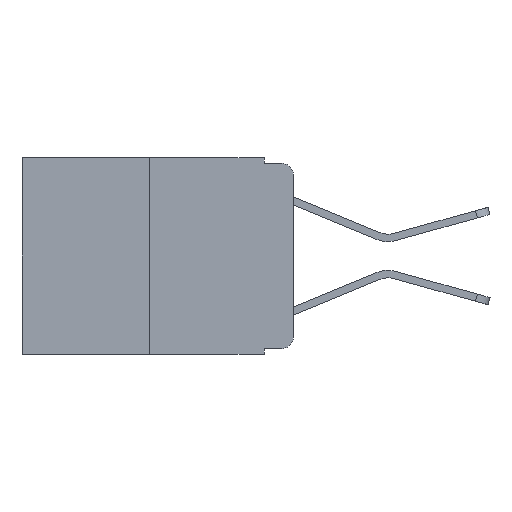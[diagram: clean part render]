
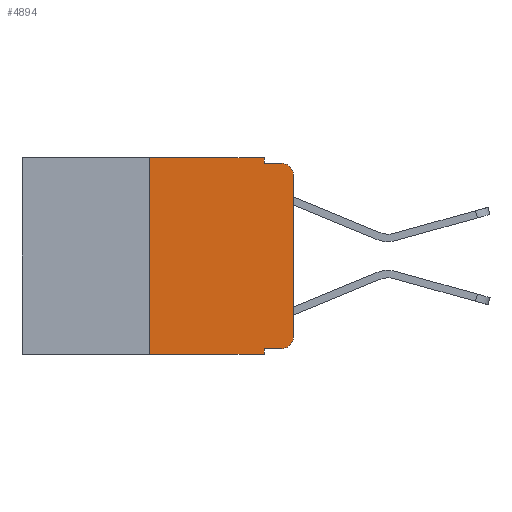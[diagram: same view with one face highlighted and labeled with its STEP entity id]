
A CAD part, left-side view. The second image highlights one B-rep face of the part: STEP entity #4894.
In plain terms, the highlighted planar face has unit normal (-1, 0, 0).
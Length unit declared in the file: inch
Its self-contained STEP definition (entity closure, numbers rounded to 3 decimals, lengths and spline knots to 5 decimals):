
#77 = CARTESIAN_POINT ( 'NONE',  ( 0., 0.02, -0.313 ) ) ;
#175 = VERTEX_POINT ( 'NONE', #5440 ) ;
#481 = FACE_OUTER_BOUND ( 'NONE', #11245, .T. ) ;
#937 = LINE ( 'NONE', #13470, #8280 ) ;
#971 = EDGE_CURVE ( 'NONE', #6619, #3720, #5943, .T. ) ;
#1068 = LINE ( 'NONE', #15789, #8590 ) ;
#1613 = ORIENTED_EDGE ( 'NONE', *, *, #971, .F. ) ;
#1691 = EDGE_CURVE ( 'NONE', #15083, #6226, #8127, .T. ) ;
#1909 = VERTEX_POINT ( 'NONE', #13209 ) ;
#2185 = ORIENTED_EDGE ( 'NONE', *, *, #8468, .T. ) ;
#2215 = CARTESIAN_POINT ( 'NONE',  ( 0., 0.051, -0.01 ) ) ;
#2357 = DIRECTION ( 'NONE',  ( 0., 0., -1. ) ) ;
#2562 = AXIS2_PLACEMENT_3D ( 'NONE', #15297, #12859, #10260 ) ;
#2727 = ORIENTED_EDGE ( 'NONE', *, *, #1691, .F. ) ;
#3245 = CIRCLE ( 'NONE', #2562, 0.02 ) ;
#3363 = ORIENTED_EDGE ( 'NONE', *, *, #11641, .T. ) ;
#3483 = DIRECTION ( 'NONE',  ( 1., 0., 0. ) ) ;
#3720 = VERTEX_POINT ( 'NONE', #12724 ) ;
#3867 = ORIENTED_EDGE ( 'NONE', *, *, #4759, .T. ) ;
#4334 = LINE ( 'NONE', #9506, #16254 ) ;
#4454 = PLANE ( 'NONE',  #15577 ) ;
#4559 = CARTESIAN_POINT ( 'NONE',  ( 0., 0.25, 0. ) ) ;
#4759 = EDGE_CURVE ( 'NONE', #8461, #175, #13996, .T. ) ;
#4894 = ADVANCED_FACE ( 'NONE', ( #481 ), #4454, .F. ) ;
#5097 = CARTESIAN_POINT ( 'NONE',  ( 0., 0.051, 0. ) ) ;
#5440 = CARTESIAN_POINT ( 'NONE',  ( 0., 0., -0.313 ) ) ;
#5709 = VECTOR ( 'NONE', #12184, 39.37008 ) ;
#5878 = LINE ( 'NONE', #9819, #7857 ) ;
#5943 = LINE ( 'NONE', #10983, #8694 ) ;
#6226 = VERTEX_POINT ( 'NONE', #2215 ) ;
#6250 = ORIENTED_EDGE ( 'NONE', *, *, #12152, .F. ) ;
#6619 = VERTEX_POINT ( 'NONE', #6769 ) ;
#6769 = CARTESIAN_POINT ( 'NONE',  ( 0., 0.051, -0.333 ) ) ;
#6835 = DIRECTION ( 'NONE',  ( 0., -1., 0. ) ) ;
#7012 = DIRECTION ( 'NONE',  ( 0., 0., -1. ) ) ;
#7691 = EDGE_CURVE ( 'NONE', #1909, #10425, #4334, .T. ) ;
#7712 = DIRECTION ( 'NONE',  ( -1., 0., 0. ) ) ;
#7757 = CARTESIAN_POINT ( 'NONE',  ( 0., 0.051, 0. ) ) ;
#7857 = VECTOR ( 'NONE', #16244, 39.37008 ) ;
#8127 = LINE ( 'NONE', #5097, #13311 ) ;
#8280 = VECTOR ( 'NONE', #9340, 39.37008 ) ;
#8325 = DIRECTION ( 'NONE',  ( 0., 0., 1. ) ) ;
#8424 = CARTESIAN_POINT ( 'NONE',  ( 0., 0.051, -0.333 ) ) ;
#8461 = VERTEX_POINT ( 'NONE', #9875 ) ;
#8468 = EDGE_CURVE ( 'NONE', #175, #11134, #5878, .T. ) ;
#8590 = VECTOR ( 'NONE', #6835, 39.37008 ) ;
#8694 = VECTOR ( 'NONE', #7012, 39.37008 ) ;
#9340 = DIRECTION ( 'NONE',  ( 0., -1., 0. ) ) ;
#9506 = CARTESIAN_POINT ( 'NONE',  ( 0., 0.25, 0. ) ) ;
#9785 = CARTESIAN_POINT ( 'NONE',  ( 0., 0.051, -0.01 ) ) ;
#9819 = CARTESIAN_POINT ( 'NONE',  ( 0., 0., 0. ) ) ;
#9843 = AXIS2_PLACEMENT_3D ( 'NONE', #77, #7712, #10406 ) ;
#9875 = CARTESIAN_POINT ( 'NONE',  ( 0., 0.02, -0.333 ) ) ;
#9995 = CARTESIAN_POINT ( 'NONE',  ( 0., 0.473, 0. ) ) ;
#10260 = DIRECTION ( 'NONE',  ( 0., 0., -1. ) ) ;
#10406 = DIRECTION ( 'NONE',  ( 0., 0., -1. ) ) ;
#10425 = VERTEX_POINT ( 'NONE', #4559 ) ;
#10691 = ORIENTED_EDGE ( 'NONE', *, *, #7691, .F. ) ;
#10983 = CARTESIAN_POINT ( 'NONE',  ( 0., 0.051, 0. ) ) ;
#10999 = CARTESIAN_POINT ( 'NONE',  ( 0., 0., -0.03 ) ) ;
#11134 = VERTEX_POINT ( 'NONE', #10999 ) ;
#11245 = EDGE_LOOP ( 'NONE', ( #2185, #15159, #6250, #2727, #11529, #10691, #3363, #1613, #13440, #3867 ) ) ;
#11529 = ORIENTED_EDGE ( 'NONE', *, *, #13740, .F. ) ;
#11641 = EDGE_CURVE ( 'NONE', #1909, #3720, #937, .T. ) ;
#12152 = EDGE_CURVE ( 'NONE', #6226, #13658, #14253, .T. ) ;
#12184 = DIRECTION ( 'NONE',  ( 0., -1., 0. ) ) ;
#12199 = EDGE_CURVE ( 'NONE', #6619, #8461, #13068, .T. ) ;
#12261 = VECTOR ( 'NONE', #16272, 39.37008 ) ;
#12724 = CARTESIAN_POINT ( 'NONE',  ( 0., 0.051, -0.343 ) ) ;
#12859 = DIRECTION ( 'NONE',  ( -1., 0., 0. ) ) ;
#13068 = LINE ( 'NONE', #8424, #12261 ) ;
#13209 = CARTESIAN_POINT ( 'NONE',  ( 0., 0.25, -0.343 ) ) ;
#13311 = VECTOR ( 'NONE', #15253, 39.37008 ) ;
#13440 = ORIENTED_EDGE ( 'NONE', *, *, #12199, .T. ) ;
#13470 = CARTESIAN_POINT ( 'NONE',  ( 0., 0.473, -0.343 ) ) ;
#13596 = EDGE_CURVE ( 'NONE', #11134, #13658, #3245, .T. ) ;
#13658 = VERTEX_POINT ( 'NONE', #15408 ) ;
#13740 = EDGE_CURVE ( 'NONE', #10425, #15083, #1068, .T. ) ;
#13996 = CIRCLE ( 'NONE', #9843, 0.02 ) ;
#14253 = LINE ( 'NONE', #9785, #5709 ) ;
#15083 = VERTEX_POINT ( 'NONE', #7757 ) ;
#15159 = ORIENTED_EDGE ( 'NONE', *, *, #13596, .T. ) ;
#15253 = DIRECTION ( 'NONE',  ( 0., 0., -1. ) ) ;
#15297 = CARTESIAN_POINT ( 'NONE',  ( 0., 0.02, -0.03 ) ) ;
#15408 = CARTESIAN_POINT ( 'NONE',  ( 0., 0.02, -0.01 ) ) ;
#15577 = AXIS2_PLACEMENT_3D ( 'NONE', #9995, #3483, #2357 ) ;
#15789 = CARTESIAN_POINT ( 'NONE',  ( 0., 0.473, 0. ) ) ;
#16244 = DIRECTION ( 'NONE',  ( 0., 0., 1. ) ) ;
#16254 = VECTOR ( 'NONE', #8325, 39.37008 ) ;
#16272 = DIRECTION ( 'NONE',  ( 0., -1., 0. ) ) ;
